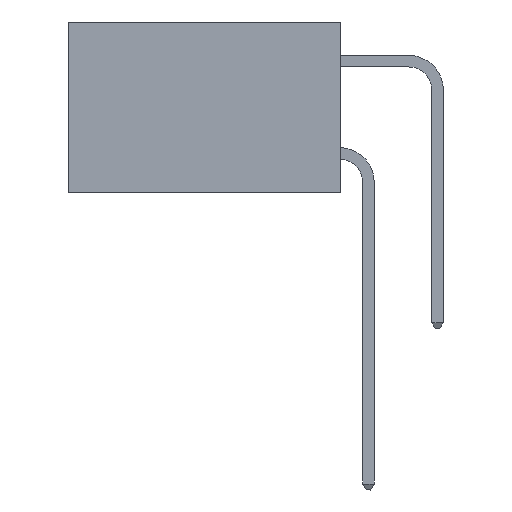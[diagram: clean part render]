
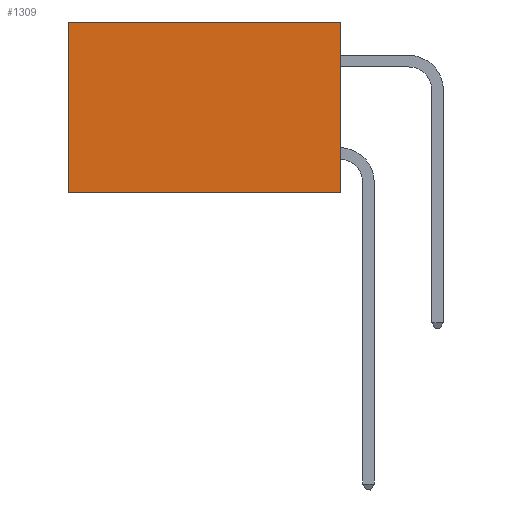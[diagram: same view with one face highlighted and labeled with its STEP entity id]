
A CAD part, left-side view. The second image highlights one B-rep face of the part: STEP entity #1309.
In plain terms, the highlighted planar face has unit normal (-1, 0, 0).
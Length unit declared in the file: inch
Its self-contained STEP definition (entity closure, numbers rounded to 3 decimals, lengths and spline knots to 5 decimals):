
#1232 = FACE_OUTER_BOUND ( 'NONE', #19890, .T. ) ;
#1306 = CARTESIAN_POINT ( 'NONE',  ( 0.277, 0.59, -0.37 ) ) ;
#1309 = ADVANCED_FACE ( 'NONE', ( #1232 ), #3381, .F. ) ;
#1465 = VERTEX_POINT ( 'NONE', #17339 ) ;
#1753 = VECTOR ( 'NONE', #22910, 39.37008 ) ;
#1911 = CARTESIAN_POINT ( 'NONE',  ( 0.277, 0., -0.37 ) ) ;
#3301 = ORIENTED_EDGE ( 'NONE', *, *, #13797, .T. ) ;
#3381 = PLANE ( 'NONE',  #14704 ) ;
#3637 = VECTOR ( 'NONE', #26022, 39.37008 ) ;
#4618 = LINE ( 'NONE', #9285, #25992 ) ;
#5278 = ORIENTED_EDGE ( 'NONE', *, *, #24144, .F. ) ;
#6881 = DIRECTION ( 'NONE',  ( 1., 0., 0. ) ) ;
#7931 = LINE ( 'NONE', #1911, #23779 ) ;
#9285 = CARTESIAN_POINT ( 'NONE',  ( 0.277, 0.59, -0.37 ) ) ;
#9805 = LINE ( 'NONE', #17780, #3637 ) ;
#9890 = ORIENTED_EDGE ( 'NONE', *, *, #12821, .F. ) ;
#10739 = CARTESIAN_POINT ( 'NONE',  ( 0.277, 0., -0.37 ) ) ;
#11415 = VERTEX_POINT ( 'NONE', #1306 ) ;
#11929 = EDGE_CURVE ( 'NONE', #1465, #23696, #12827, .T. ) ;
#12821 = EDGE_CURVE ( 'NONE', #1465, #21428, #7931, .T. ) ;
#12827 = LINE ( 'NONE', #23572, #1753 ) ;
#13797 = EDGE_CURVE ( 'NONE', #23696, #11415, #4618, .T. ) ;
#14704 = AXIS2_PLACEMENT_3D ( 'NONE', #24173, #6881, #24024 ) ;
#17339 = CARTESIAN_POINT ( 'NONE',  ( 0.277, 0., 0. ) ) ;
#17780 = CARTESIAN_POINT ( 'NONE',  ( 0.277, 0., -0.37 ) ) ;
#18520 = DIRECTION ( 'NONE',  ( 0., 0., -1. ) ) ;
#18656 = ORIENTED_EDGE ( 'NONE', *, *, #11929, .T. ) ;
#19890 = EDGE_LOOP ( 'NONE', ( #3301, #5278, #9890, #18656 ) ) ;
#21428 = VERTEX_POINT ( 'NONE', #10739 ) ;
#22910 = DIRECTION ( 'NONE',  ( 0., 1., 0. ) ) ;
#23572 = CARTESIAN_POINT ( 'NONE',  ( 0.277, 0., 0. ) ) ;
#23696 = VERTEX_POINT ( 'NONE', #26785 ) ;
#23725 = DIRECTION ( 'NONE',  ( 0., 0., -1. ) ) ;
#23779 = VECTOR ( 'NONE', #18520, 39.37008 ) ;
#24024 = DIRECTION ( 'NONE',  ( 0., 0., -1. ) ) ;
#24144 = EDGE_CURVE ( 'NONE', #21428, #11415, #9805, .T. ) ;
#24173 = CARTESIAN_POINT ( 'NONE',  ( 0.277, 0., -0.37 ) ) ;
#25992 = VECTOR ( 'NONE', #23725, 39.37008 ) ;
#26022 = DIRECTION ( 'NONE',  ( 0., 1., 0. ) ) ;
#26785 = CARTESIAN_POINT ( 'NONE',  ( 0.277, 0.59, 0. ) ) ;
